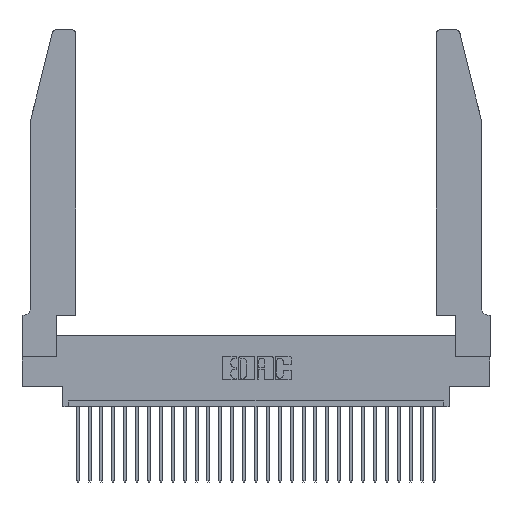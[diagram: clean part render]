
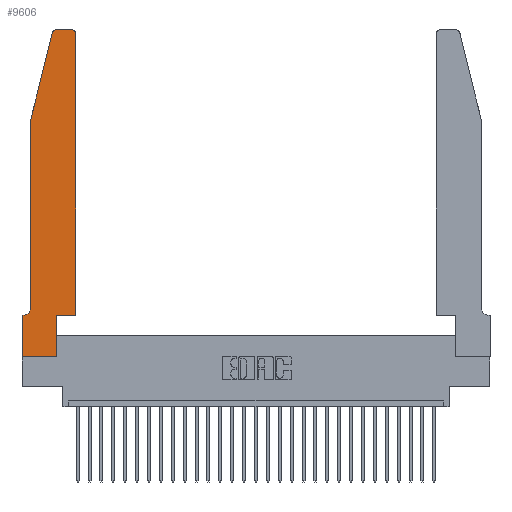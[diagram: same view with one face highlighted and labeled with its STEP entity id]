
A CAD part, top view. The second image highlights one B-rep face of the part: STEP entity #9606.
In plain terms, the highlighted planar face has unit normal (0, 0, 1).
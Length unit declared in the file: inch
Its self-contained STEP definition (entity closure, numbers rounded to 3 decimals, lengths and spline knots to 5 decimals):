
#84 = VERTEX_POINT ( 'NONE', #3067 ) ;
#247 = EDGE_CURVE ( 'NONE', #28621, #17095, #16655, .T. ) ;
#328 = VERTEX_POINT ( 'NONE', #15332 ) ;
#643 = ORIENTED_EDGE ( 'NONE', *, *, #26793, .T. ) ;
#760 = AXIS2_PLACEMENT_3D ( 'NONE', #27942, #7412, #9422 ) ;
#764 = ORIENTED_EDGE ( 'NONE', *, *, #23410, .T. ) ;
#830 = AXIS2_PLACEMENT_3D ( 'NONE', #22087, #9373, #18318 ) ;
#1834 = LINE ( 'NONE', #12101, #25869 ) ;
#2007 = VECTOR ( 'NONE', #10176, 39.37008 ) ;
#2365 = VERTEX_POINT ( 'NONE', #13619 ) ;
#2634 = VECTOR ( 'NONE', #13339, 39.37008 ) ;
#2786 = ORIENTED_EDGE ( 'NONE', *, *, #21665, .T. ) ;
#2860 = VECTOR ( 'NONE', #13542, 39.37008 ) ;
#3064 = ORIENTED_EDGE ( 'NONE', *, *, #21358, .T. ) ;
#3067 = CARTESIAN_POINT ( 'NONE',  ( 0.0055, 0.35, 0.37 ) ) ;
#3666 = CARTESIAN_POINT ( 'NONE',  ( 0.0755, 0.35, 0.37 ) ) ;
#3725 = CARTESIAN_POINT ( 'NONE',  ( 0.2865, 0.35, 0.37 ) ) ;
#4122 = CARTESIAN_POINT ( 'NONE',  ( 0.2605, 2.75, 0.37 ) ) ;
#4225 = DIRECTION ( 'NONE',  ( 0., 0., 1. ) ) ;
#4825 = ORIENTED_EDGE ( 'NONE', *, *, #18448, .T. ) ;
#5102 = EDGE_CURVE ( 'NONE', #22324, #28621, #10782, .T. ) ;
#5341 = DIRECTION ( 'NONE',  ( 1., 0., 0. ) ) ;
#5509 = FACE_OUTER_BOUND ( 'NONE', #20103, .T. ) ;
#5714 = CARTESIAN_POINT ( 'NONE',  ( 0.4505, 0.35, 0.37 ) ) ;
#5929 = CARTESIAN_POINT ( 'NONE',  ( 0.4505, 2.72, 0.37 ) ) ;
#6674 = VERTEX_POINT ( 'NONE', #15161 ) ;
#7412 = DIRECTION ( 'NONE',  ( 0., 0., 1. ) ) ;
#7845 = ORIENTED_EDGE ( 'NONE', *, *, #16064, .T. ) ;
#8309 = DIRECTION ( 'NONE',  ( -1., 0., 0. ) ) ;
#8756 = CARTESIAN_POINT ( 'NONE',  ( 0.4205, 2.75, 0.37 ) ) ;
#8768 = AXIS2_PLACEMENT_3D ( 'NONE', #14619, #19466, #5341 ) ;
#9373 = DIRECTION ( 'NONE',  ( 0., 0., -1. ) ) ;
#9422 = DIRECTION ( 'NONE',  ( 1., 0., 0. ) ) ;
#9441 = LINE ( 'NONE', #22285, #18409 ) ;
#9581 = CIRCLE ( 'NONE', #8768, 0.03 ) ;
#9606 = ADVANCED_FACE ( 'NONE', ( #5509 ), #21097, .T. ) ;
#10176 = DIRECTION ( 'NONE',  ( 1., 0., 0. ) ) ;
#10529 = VERTEX_POINT ( 'NONE', #8756 ) ;
#10782 = LINE ( 'NONE', #16039, #2860 ) ;
#10857 = EDGE_CURVE ( 'NONE', #22266, #17266, #9581, .T. ) ;
#11145 = VECTOR ( 'NONE', #8309, 39.37008 ) ;
#11359 = CARTESIAN_POINT ( 'NONE',  ( 0.0755, 2., 0.37 ) ) ;
#12101 = CARTESIAN_POINT ( 'NONE',  ( 0.2865, 0.35, 0.37 ) ) ;
#12471 = CARTESIAN_POINT ( 'NONE',  ( 0., 0., 0.37 ) ) ;
#12572 = LINE ( 'NONE', #3666, #11145 ) ;
#12657 = VERTEX_POINT ( 'NONE', #21715 ) ;
#12844 = ORIENTED_EDGE ( 'NONE', *, *, #5102, .T. ) ;
#13339 = DIRECTION ( 'NONE',  ( 0., 1., 0. ) ) ;
#13542 = DIRECTION ( 'NONE',  ( 1., 0., 0. ) ) ;
#13619 = CARTESIAN_POINT ( 'NONE',  ( 0.2865, 0., 0.37 ) ) ;
#13778 = DIRECTION ( 'NONE',  ( 0., -1., 0. ) ) ;
#13785 = DIRECTION ( 'NONE',  ( -0.239, -0.971, 0. ) ) ;
#14445 = DIRECTION ( 'NONE',  ( 0., 1., 0. ) ) ;
#14619 = CARTESIAN_POINT ( 'NONE',  ( 0.284, 2.72, 0.37 ) ) ;
#14828 = CIRCLE ( 'NONE', #16974, 0.03 ) ;
#15161 = CARTESIAN_POINT ( 'NONE',  ( 0., 0., 0.37 ) ) ;
#15239 = DIRECTION ( 'NONE',  ( 0., -1., 0. ) ) ;
#15332 = CARTESIAN_POINT ( 'NONE',  ( 0.0755, 2., 0.37 ) ) ;
#15531 = DIRECTION ( 'NONE',  ( 1., 0., 0. ) ) ;
#15786 = EDGE_CURVE ( 'NONE', #328, #12657, #22631, .T. ) ;
#16039 = CARTESIAN_POINT ( 'NONE',  ( 0.4505, 0.35, 0.37 ) ) ;
#16064 = EDGE_CURVE ( 'NONE', #20987, #6674, #9441, .T. ) ;
#16361 = ORIENTED_EDGE ( 'NONE', *, *, #10857, .T. ) ;
#16655 = LINE ( 'NONE', #24485, #2634 ) ;
#16974 = AXIS2_PLACEMENT_3D ( 'NONE', #22571, #4225, #15531 ) ;
#17095 = VERTEX_POINT ( 'NONE', #5929 ) ;
#17266 = VERTEX_POINT ( 'NONE', #25954 ) ;
#18024 = CARTESIAN_POINT ( 'NONE',  ( 0., 0.35, 0.37 ) ) ;
#18318 = DIRECTION ( 'NONE',  ( -1., 0., 0. ) ) ;
#18409 = VECTOR ( 'NONE', #15239, 39.37008 ) ;
#18448 = EDGE_CURVE ( 'NONE', #2365, #22324, #1834, .T. ) ;
#18549 = EDGE_CURVE ( 'NONE', #17095, #10529, #14828, .T. ) ;
#18679 = ORIENTED_EDGE ( 'NONE', *, *, #26218, .T. ) ;
#19466 = DIRECTION ( 'NONE',  ( 0., 0., 1. ) ) ;
#20103 = EDGE_LOOP ( 'NONE', ( #2786, #16361, #643, #28638, #3064, #764, #7845, #18679, #4825, #12844, #28540, #22095 ) ) ;
#20364 = DIRECTION ( 'NONE',  ( -1., 0., 0. ) ) ;
#20987 = VERTEX_POINT ( 'NONE', #18024 ) ;
#21097 = PLANE ( 'NONE',  #760 ) ;
#21358 = EDGE_CURVE ( 'NONE', #12657, #84, #23674, .T. ) ;
#21665 = EDGE_CURVE ( 'NONE', #10529, #22266, #28598, .T. ) ;
#21715 = CARTESIAN_POINT ( 'NONE',  ( 0.0755, 0.42, 0.37 ) ) ;
#22087 = CARTESIAN_POINT ( 'NONE',  ( 0.0055, 0.42, 0.37 ) ) ;
#22095 = ORIENTED_EDGE ( 'NONE', *, *, #18549, .T. ) ;
#22266 = VERTEX_POINT ( 'NONE', #26319 ) ;
#22285 = CARTESIAN_POINT ( 'NONE',  ( 0., 0., 0.37 ) ) ;
#22324 = VERTEX_POINT ( 'NONE', #3725 ) ;
#22571 = CARTESIAN_POINT ( 'NONE',  ( 0.4205, 2.72, 0.37 ) ) ;
#22597 = VECTOR ( 'NONE', #20364, 39.37008 ) ;
#22631 = LINE ( 'NONE', #22934, #23326 ) ;
#22934 = CARTESIAN_POINT ( 'NONE',  ( 0.0755, 2., 0.37 ) ) ;
#23326 = VECTOR ( 'NONE', #13778, 39.37008 ) ;
#23410 = EDGE_CURVE ( 'NONE', #84, #20987, #12572, .T. ) ;
#23674 = CIRCLE ( 'NONE', #830, 0.07 ) ;
#24485 = CARTESIAN_POINT ( 'NONE',  ( 0.4505, 0.35, 0.37 ) ) ;
#25610 = VECTOR ( 'NONE', #13785, 39.37008 ) ;
#25869 = VECTOR ( 'NONE', #14445, 39.37008 ) ;
#25954 = CARTESIAN_POINT ( 'NONE',  ( 0.25487, 2.72718, 0.37 ) ) ;
#26218 = EDGE_CURVE ( 'NONE', #6674, #2365, #27186, .T. ) ;
#26319 = CARTESIAN_POINT ( 'NONE',  ( 0.284, 2.75, 0.37 ) ) ;
#26793 = EDGE_CURVE ( 'NONE', #17266, #328, #28447, .T. ) ;
#27186 = LINE ( 'NONE', #12471, #2007 ) ;
#27942 = CARTESIAN_POINT ( 'NONE',  ( 0., 0.35, 0.37 ) ) ;
#28447 = LINE ( 'NONE', #11359, #25610 ) ;
#28540 = ORIENTED_EDGE ( 'NONE', *, *, #247, .T. ) ;
#28598 = LINE ( 'NONE', #4122, #22597 ) ;
#28621 = VERTEX_POINT ( 'NONE', #5714 ) ;
#28638 = ORIENTED_EDGE ( 'NONE', *, *, #15786, .T. ) ;
